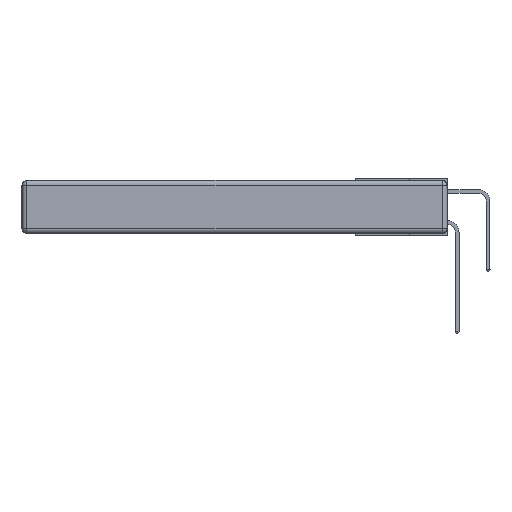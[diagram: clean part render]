
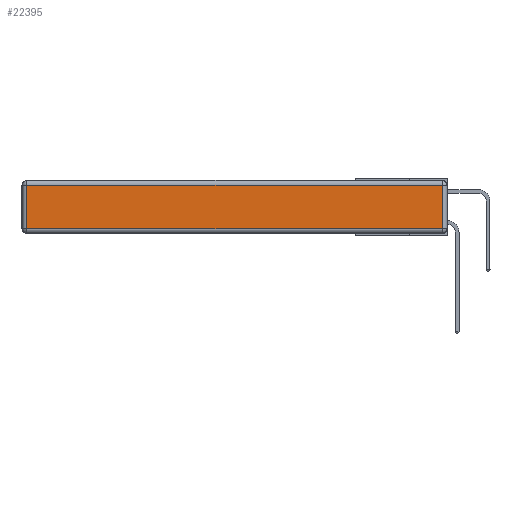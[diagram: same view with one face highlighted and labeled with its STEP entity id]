
A CAD part, left-side view. The second image highlights one B-rep face of the part: STEP entity #22395.
In plain terms, the highlighted planar face has unit normal (-1, 0, 0).
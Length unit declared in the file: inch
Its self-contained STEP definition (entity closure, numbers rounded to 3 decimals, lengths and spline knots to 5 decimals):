
#1138 = EDGE_LOOP ( 'NONE', ( #32638, #4521, #26720, #13669 ) ) ;
#2386 = VECTOR ( 'NONE', #2794, 39.37008 ) ;
#2794 = DIRECTION ( 'NONE',  ( 0., 1., 0. ) ) ;
#2930 = CARTESIAN_POINT ( 'NONE',  ( 0., 0.03, -0.03 ) ) ;
#3548 = VERTEX_POINT ( 'NONE', #11550 ) ;
#4435 = VERTEX_POINT ( 'NONE', #15284 ) ;
#4521 = ORIENTED_EDGE ( 'NONE', *, *, #33525, .T. ) ;
#4928 = DIRECTION ( 'NONE',  ( 0., -1., 0. ) ) ;
#5099 = DIRECTION ( 'NONE',  ( 0., 0., 1. ) ) ;
#6614 = AXIS2_PLACEMENT_3D ( 'NONE', #20777, #13019, #5099 ) ;
#7207 = CARTESIAN_POINT ( 'NONE',  ( 0., 0., -0.313 ) ) ;
#8171 = VECTOR ( 'NONE', #33315, 39.37008 ) ;
#8258 = VERTEX_POINT ( 'NONE', #30227 ) ;
#8373 = DIRECTION ( 'NONE',  ( 0., 0., -1. ) ) ;
#8718 = LINE ( 'NONE', #7207, #15249 ) ;
#8796 = EDGE_CURVE ( 'NONE', #8258, #3548, #25729, .T. ) ;
#11550 = CARTESIAN_POINT ( 'NONE',  ( 0., 2.72, -0.313 ) ) ;
#13019 = DIRECTION ( 'NONE',  ( -1., 0., 0. ) ) ;
#13312 = EDGE_CURVE ( 'NONE', #3548, #4435, #8718, .T. ) ;
#13669 = ORIENTED_EDGE ( 'NONE', *, *, #8796, .T. ) ;
#15249 = VECTOR ( 'NONE', #4928, 39.37008 ) ;
#15284 = CARTESIAN_POINT ( 'NONE',  ( 0., 0.03, -0.313 ) ) ;
#16331 = LINE ( 'NONE', #20536, #2386 ) ;
#16372 = FACE_OUTER_BOUND ( 'NONE', #1138, .T. ) ;
#20536 = CARTESIAN_POINT ( 'NONE',  ( 0., 2.75, -0.03 ) ) ;
#20777 = CARTESIAN_POINT ( 'NONE',  ( 0., 0., -0.343 ) ) ;
#20992 = EDGE_CURVE ( 'NONE', #28175, #8258, #16331, .T. ) ;
#21407 = CARTESIAN_POINT ( 'NONE',  ( 0., 2.72, -0.343 ) ) ;
#22395 = ADVANCED_FACE ( 'NONE', ( #16372 ), #33788, .T. ) ;
#25729 = LINE ( 'NONE', #21407, #29752 ) ;
#26720 = ORIENTED_EDGE ( 'NONE', *, *, #20992, .T. ) ;
#28175 = VERTEX_POINT ( 'NONE', #2930 ) ;
#29752 = VECTOR ( 'NONE', #8373, 39.37008 ) ;
#29854 = LINE ( 'NONE', #30563, #8171 ) ;
#30227 = CARTESIAN_POINT ( 'NONE',  ( 0., 2.72, -0.03 ) ) ;
#30563 = CARTESIAN_POINT ( 'NONE',  ( 0., 0.03, -0.343 ) ) ;
#32638 = ORIENTED_EDGE ( 'NONE', *, *, #13312, .T. ) ;
#33315 = DIRECTION ( 'NONE',  ( 0., 0., 1. ) ) ;
#33525 = EDGE_CURVE ( 'NONE', #4435, #28175, #29854, .T. ) ;
#33788 = PLANE ( 'NONE',  #6614 ) ;
